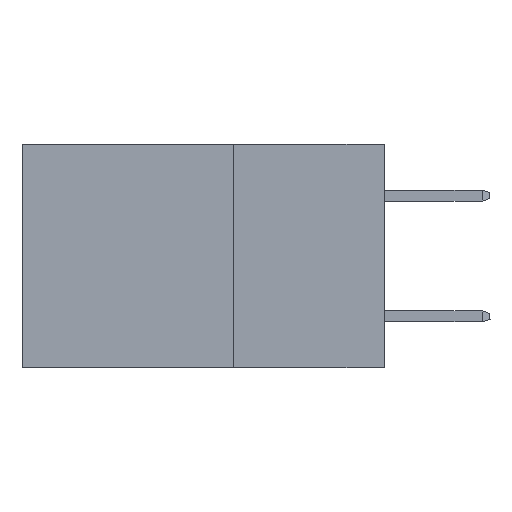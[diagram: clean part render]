
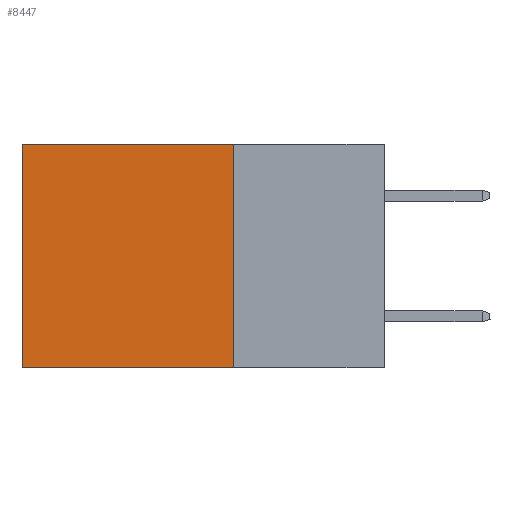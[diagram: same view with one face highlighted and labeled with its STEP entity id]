
A CAD part, left-side view. The second image highlights one B-rep face of the part: STEP entity #8447.
In plain terms, the highlighted planar face has unit normal (-1, 0, 0).
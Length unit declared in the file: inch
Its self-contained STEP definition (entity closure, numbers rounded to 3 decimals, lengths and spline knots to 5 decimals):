
#3 = PLANE ( 'NONE',  #5609 ) ;
#484 = EDGE_CURVE ( 'NONE', #18037, #11986, #17675, .T. ) ;
#1588 = CARTESIAN_POINT ( 'NONE',  ( 0.2615, 0.25, -0.37 ) ) ;
#1897 = EDGE_CURVE ( 'NONE', #11986, #19704, #18794, .T. ) ;
#2857 = EDGE_CURVE ( 'NONE', #18037, #3642, #13804, .T. ) ;
#3642 = VERTEX_POINT ( 'NONE', #15059 ) ;
#4493 = EDGE_CURVE ( 'NONE', #3642, #19704, #12261, .T. ) ;
#4521 = CARTESIAN_POINT ( 'NONE',  ( 0.2615, 0.6, -0.37 ) ) ;
#4705 = DIRECTION ( 'NONE',  ( 0., 0., -1. ) ) ;
#5440 = ORIENTED_EDGE ( 'NONE', *, *, #1897, .T. ) ;
#5609 = AXIS2_PLACEMENT_3D ( 'NONE', #1588, #14013, #4705 ) ;
#5624 = CARTESIAN_POINT ( 'NONE',  ( 0.2615, 0.25, -0.37 ) ) ;
#5648 = DIRECTION ( 'NONE',  ( 0., 1., 0. ) ) ;
#6344 = DIRECTION ( 'NONE',  ( 0., 0., -1. ) ) ;
#7221 = FACE_OUTER_BOUND ( 'NONE', #16790, .T. ) ;
#7388 = ORIENTED_EDGE ( 'NONE', *, *, #484, .T. ) ;
#8115 = VECTOR ( 'NONE', #5648, 39.37008 ) ;
#8447 = ADVANCED_FACE ( 'NONE', ( #7221 ), #3, .F. ) ;
#8526 = VECTOR ( 'NONE', #6344, 39.37008 ) ;
#9255 = ORIENTED_EDGE ( 'NONE', *, *, #2857, .F. ) ;
#9724 = VECTOR ( 'NONE', #11305, 39.37008 ) ;
#9926 = CARTESIAN_POINT ( 'NONE',  ( 0.2615, 0.6, -0.37 ) ) ;
#11305 = DIRECTION ( 'NONE',  ( 0., 0., -1. ) ) ;
#11986 = VERTEX_POINT ( 'NONE', #16788 ) ;
#12230 = CARTESIAN_POINT ( 'NONE',  ( 0.2615, 0.25, -0.37 ) ) ;
#12261 = LINE ( 'NONE', #5624, #8115 ) ;
#13804 = LINE ( 'NONE', #12230, #9724 ) ;
#14013 = DIRECTION ( 'NONE',  ( 1., 0., 0. ) ) ;
#14260 = CARTESIAN_POINT ( 'NONE',  ( 0.2615, 0.25, 0. ) ) ;
#15059 = CARTESIAN_POINT ( 'NONE',  ( 0.2615, 0.25, -0.37 ) ) ;
#16788 = CARTESIAN_POINT ( 'NONE',  ( 0.2615, 0.6, 0. ) ) ;
#16790 = EDGE_LOOP ( 'NONE', ( #5440, #19649, #9255, #7388 ) ) ;
#17219 = VECTOR ( 'NONE', #19176, 39.37008 ) ;
#17675 = LINE ( 'NONE', #14260, #17219 ) ;
#18037 = VERTEX_POINT ( 'NONE', #18500 ) ;
#18500 = CARTESIAN_POINT ( 'NONE',  ( 0.2615, 0.25, 0. ) ) ;
#18794 = LINE ( 'NONE', #4521, #8526 ) ;
#19176 = DIRECTION ( 'NONE',  ( 0., 1., 0. ) ) ;
#19649 = ORIENTED_EDGE ( 'NONE', *, *, #4493, .F. ) ;
#19704 = VERTEX_POINT ( 'NONE', #9926 ) ;
